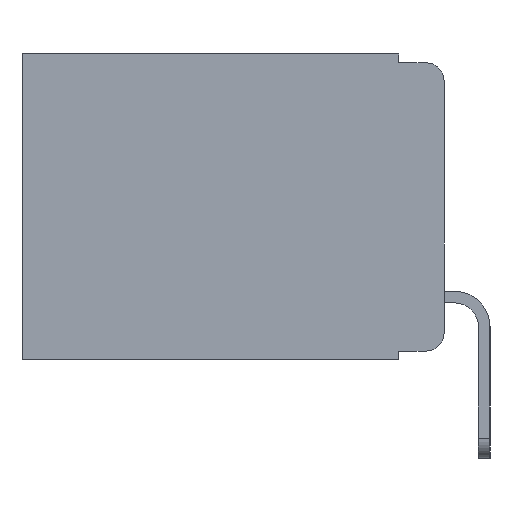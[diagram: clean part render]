
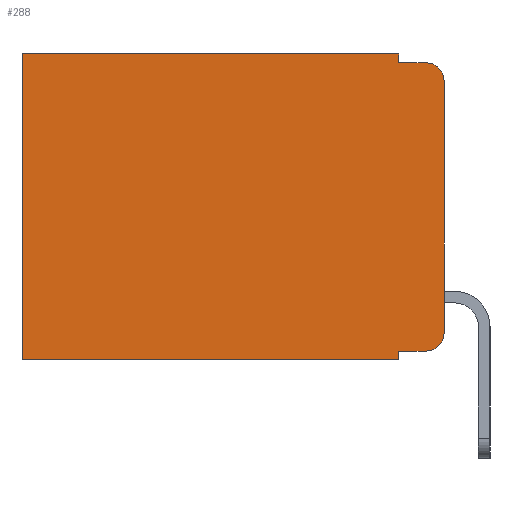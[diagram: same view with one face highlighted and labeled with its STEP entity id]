
A CAD part, left-side view. The second image highlights one B-rep face of the part: STEP entity #288.
In plain terms, the highlighted planar face has unit normal (-1, 0, 0).
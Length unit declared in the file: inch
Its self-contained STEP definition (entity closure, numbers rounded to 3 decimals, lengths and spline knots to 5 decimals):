
#288 = ADVANCED_FACE ( 'NONE', ( #6342 ), #5572, .F. ) ;
#534 = ORIENTED_EDGE ( 'NONE', *, *, #11708, .T. ) ;
#584 = ORIENTED_EDGE ( 'NONE', *, *, #10569, .F. ) ;
#708 = VECTOR ( 'NONE', #6620, 39.37008 ) ;
#901 = ORIENTED_EDGE ( 'NONE', *, *, #10432, .T. ) ;
#1149 = VECTOR ( 'NONE', #12127, 39.37008 ) ;
#1177 = CARTESIAN_POINT ( 'NONE',  ( 0.298, 0.02, -0.313 ) ) ;
#1499 = ORIENTED_EDGE ( 'NONE', *, *, #10822, .F. ) ;
#1581 = LINE ( 'NONE', #8297, #1149 ) ;
#2031 = ORIENTED_EDGE ( 'NONE', *, *, #10493, .T. ) ;
#2126 = EDGE_LOOP ( 'NONE', ( #584, #2298, #2246, #3720, #534, #2031, #1499, #3973, #3374, #901 ) ) ;
#2132 = VERTEX_POINT ( 'NONE', #10724 ) ;
#2177 = CARTESIAN_POINT ( 'NONE',  ( 0.298, 0.473, 0. ) ) ;
#2246 = ORIENTED_EDGE ( 'NONE', *, *, #10509, .F. ) ;
#2298 = ORIENTED_EDGE ( 'NONE', *, *, #10542, .T. ) ;
#2432 = VERTEX_POINT ( 'NONE', #7259 ) ;
#2476 = DIRECTION ( 'NONE',  ( 0., 0., -1. ) ) ;
#2613 = VERTEX_POINT ( 'NONE', #6989 ) ;
#2861 = DIRECTION ( 'NONE',  ( 0., 0., -1. ) ) ;
#3221 = VERTEX_POINT ( 'NONE', #8340 ) ;
#3374 = ORIENTED_EDGE ( 'NONE', *, *, #10446, .T. ) ;
#3693 = AXIS2_PLACEMENT_3D ( 'NONE', #4557, #5679, #2861 ) ;
#3720 = ORIENTED_EDGE ( 'NONE', *, *, #10507, .F. ) ;
#3874 = VERTEX_POINT ( 'NONE', #4599 ) ;
#3973 = ORIENTED_EDGE ( 'NONE', *, *, #10470, .F. ) ;
#4557 = CARTESIAN_POINT ( 'NONE',  ( 0.298, 0., 0. ) ) ;
#4599 = CARTESIAN_POINT ( 'NONE',  ( 0.298, 0.02, -0.333 ) ) ;
#4642 = LINE ( 'NONE', #4709, #6831 ) ;
#4709 = CARTESIAN_POINT ( 'NONE',  ( 0.298, 0.051, 0. ) ) ;
#4750 = AXIS2_PLACEMENT_3D ( 'NONE', #10739, #5800, #11473 ) ;
#4774 = LINE ( 'NONE', #6639, #6658 ) ;
#4888 = VERTEX_POINT ( 'NONE', #8796 ) ;
#4954 = VERTEX_POINT ( 'NONE', #2177 ) ;
#5198 = CARTESIAN_POINT ( 'NONE',  ( 0.298, 0., -0.343 ) ) ;
#5572 = PLANE ( 'NONE',  #3693 ) ;
#5679 = DIRECTION ( 'NONE',  ( 1., 0., 0. ) ) ;
#5753 = CARTESIAN_POINT ( 'NONE',  ( 0.298, 0.051, -0.01 ) ) ;
#5800 = DIRECTION ( 'NONE',  ( -1., 0., 0. ) ) ;
#6025 = VECTOR ( 'NONE', #8362, 39.37008 ) ;
#6150 = LINE ( 'NONE', #5198, #10062 ) ;
#6282 = CIRCLE ( 'NONE', #4750, 0.02 ) ;
#6342 = FACE_OUTER_BOUND ( 'NONE', #2126, .T. ) ;
#6503 = CARTESIAN_POINT ( 'NONE',  ( 0.298, 0.051, -0.333 ) ) ;
#6546 = VECTOR ( 'NONE', #10705, 39.37008 ) ;
#6620 = DIRECTION ( 'NONE',  ( 0., -1., 0. ) ) ;
#6639 = CARTESIAN_POINT ( 'NONE',  ( 0.298, 0., 0. ) ) ;
#6658 = VECTOR ( 'NONE', #12144, 39.37008 ) ;
#6661 = CARTESIAN_POINT ( 'NONE',  ( 0.298, 0., 0. ) ) ;
#6718 = CARTESIAN_POINT ( 'NONE',  ( 0.298, 0.473, -0.343 ) ) ;
#6831 = VECTOR ( 'NONE', #9898, 39.37008 ) ;
#6989 = CARTESIAN_POINT ( 'NONE',  ( 0.298, 0.051, -0.343 ) ) ;
#7094 = LINE ( 'NONE', #6503, #11105 ) ;
#7259 = CARTESIAN_POINT ( 'NONE',  ( 0.298, 0.02, -0.01 ) ) ;
#7988 = VERTEX_POINT ( 'NONE', #10908 ) ;
#8264 = DIRECTION ( 'NONE',  ( -1., 0., 0. ) ) ;
#8279 = LINE ( 'NONE', #6661, #6025 ) ;
#8297 = CARTESIAN_POINT ( 'NONE',  ( 0.298, 0.473, 0. ) ) ;
#8340 = CARTESIAN_POINT ( 'NONE',  ( 0.298, 0., -0.313 ) ) ;
#8362 = DIRECTION ( 'NONE',  ( 0., 0., -1. ) ) ;
#8796 = CARTESIAN_POINT ( 'NONE',  ( 0.298, 0.051, 0. ) ) ;
#8823 = LINE ( 'NONE', #5753, #708 ) ;
#8902 = AXIS2_PLACEMENT_3D ( 'NONE', #1177, #8264, #2476 ) ;
#9315 = VERTEX_POINT ( 'NONE', #6718 ) ;
#9818 = CIRCLE ( 'NONE', #8902, 0.02 ) ;
#9898 = DIRECTION ( 'NONE',  ( 0., 0., -1. ) ) ;
#9948 = CARTESIAN_POINT ( 'NONE',  ( 0.298, 0.051, 0. ) ) ;
#10062 = VECTOR ( 'NONE', #10993, 39.37008 ) ;
#10432 = EDGE_CURVE ( 'NONE', #3874, #3221, #9818, .T. ) ;
#10446 = EDGE_CURVE ( 'NONE', #2132, #3874, #7094, .T. ) ;
#10470 = EDGE_CURVE ( 'NONE', #2132, #2613, #4642, .T. ) ;
#10493 = EDGE_CURVE ( 'NONE', #4954, #9315, #1581, .T. ) ;
#10507 = EDGE_CURVE ( 'NONE', #4888, #7988, #10871, .T. ) ;
#10509 = EDGE_CURVE ( 'NONE', #7988, #2432, #8823, .T. ) ;
#10542 = EDGE_CURVE ( 'NONE', #10567, #2432, #6282, .T. ) ;
#10567 = VERTEX_POINT ( 'NONE', #12180 ) ;
#10569 = EDGE_CURVE ( 'NONE', #10567, #3221, #8279, .T. ) ;
#10705 = DIRECTION ( 'NONE',  ( 0., 0., -1. ) ) ;
#10724 = CARTESIAN_POINT ( 'NONE',  ( 0.298, 0.051, -0.333 ) ) ;
#10739 = CARTESIAN_POINT ( 'NONE',  ( 0.298, 0.02, -0.03 ) ) ;
#10822 = EDGE_CURVE ( 'NONE', #2613, #9315, #6150, .T. ) ;
#10871 = LINE ( 'NONE', #9948, #6546 ) ;
#10908 = CARTESIAN_POINT ( 'NONE',  ( 0.298, 0.051, -0.01 ) ) ;
#10993 = DIRECTION ( 'NONE',  ( 0., 1., 0. ) ) ;
#11105 = VECTOR ( 'NONE', #11371, 39.37008 ) ;
#11371 = DIRECTION ( 'NONE',  ( 0., -1., 0. ) ) ;
#11473 = DIRECTION ( 'NONE',  ( 0., 0., -1. ) ) ;
#11708 = EDGE_CURVE ( 'NONE', #4888, #4954, #4774, .T. ) ;
#12127 = DIRECTION ( 'NONE',  ( 0., 0., -1. ) ) ;
#12144 = DIRECTION ( 'NONE',  ( 0., 1., 0. ) ) ;
#12180 = CARTESIAN_POINT ( 'NONE',  ( 0.298, 0., -0.03 ) ) ;
